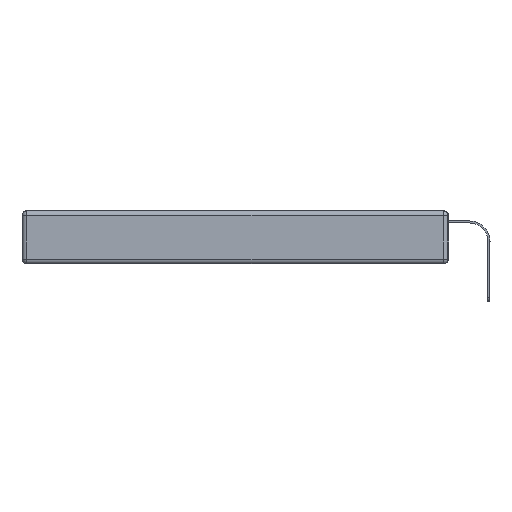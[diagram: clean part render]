
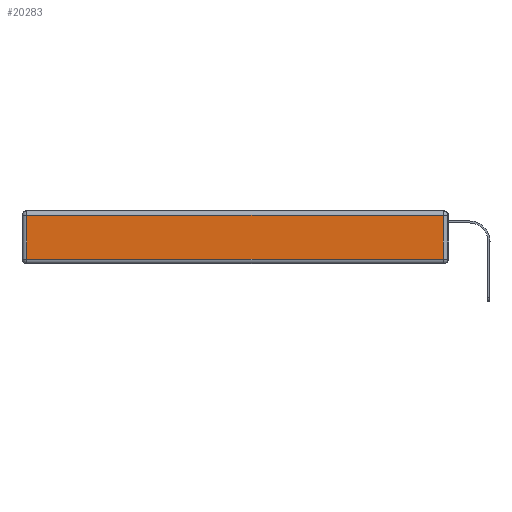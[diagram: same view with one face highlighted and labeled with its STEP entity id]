
A CAD part, left-side view. The second image highlights one B-rep face of the part: STEP entity #20283.
In plain terms, the highlighted planar face has unit normal (-1, 0, 0).
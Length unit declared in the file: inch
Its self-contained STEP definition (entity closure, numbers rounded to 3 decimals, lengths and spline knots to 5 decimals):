
#1440 = ORIENTED_EDGE ( 'NONE', *, *, #4398, .T. ) ;
#2004 = CARTESIAN_POINT ( 'NONE',  ( 0., 0.03, -0.03 ) ) ;
#2125 = VERTEX_POINT ( 'NONE', #2004 ) ;
#2507 = EDGE_CURVE ( 'NONE', #13487, #12943, #13361, .T. ) ;
#2826 = ORIENTED_EDGE ( 'NONE', *, *, #2507, .T. ) ;
#3901 = CARTESIAN_POINT ( 'NONE',  ( 0., 2.72, -0.343 ) ) ;
#3906 = VERTEX_POINT ( 'NONE', #17260 ) ;
#4398 = EDGE_CURVE ( 'NONE', #3906, #2125, #18825, .T. ) ;
#4701 = DIRECTION ( 'NONE',  ( 0., 0., 1. ) ) ;
#6167 = EDGE_LOOP ( 'NONE', ( #6197, #1440, #10350, #2826 ) ) ;
#6171 = LINE ( 'NONE', #14358, #8982 ) ;
#6197 = ORIENTED_EDGE ( 'NONE', *, *, #20880, .T. ) ;
#6198 = CARTESIAN_POINT ( 'NONE',  ( 0., 0., -0.343 ) ) ;
#7205 = DIRECTION ( 'NONE',  ( 0., -1., 0. ) ) ;
#8725 = CARTESIAN_POINT ( 'NONE',  ( 0., 0., -0.313 ) ) ;
#8902 = CARTESIAN_POINT ( 'NONE',  ( 0., 2.72, -0.03 ) ) ;
#8982 = VECTOR ( 'NONE', #14465, 39.37008 ) ;
#10042 = VECTOR ( 'NONE', #12471, 39.37008 ) ;
#10350 = ORIENTED_EDGE ( 'NONE', *, *, #18829, .T. ) ;
#10643 = CARTESIAN_POINT ( 'NONE',  ( 0., 0.03, -0.343 ) ) ;
#11172 = PLANE ( 'NONE',  #18253 ) ;
#12042 = CARTESIAN_POINT ( 'NONE',  ( 0., 2.72, -0.313 ) ) ;
#12471 = DIRECTION ( 'NONE',  ( 0., 0., 1. ) ) ;
#12766 = FACE_OUTER_BOUND ( 'NONE', #6167, .T. ) ;
#12943 = VERTEX_POINT ( 'NONE', #12042 ) ;
#13342 = VECTOR ( 'NONE', #15405, 39.37008 ) ;
#13361 = LINE ( 'NONE', #3901, #13342 ) ;
#13487 = VERTEX_POINT ( 'NONE', #8902 ) ;
#14358 = CARTESIAN_POINT ( 'NONE',  ( 0., 2.75, -0.03 ) ) ;
#14465 = DIRECTION ( 'NONE',  ( 0., 1., 0. ) ) ;
#15177 = VECTOR ( 'NONE', #7205, 39.37008 ) ;
#15405 = DIRECTION ( 'NONE',  ( 0., 0., -1. ) ) ;
#17260 = CARTESIAN_POINT ( 'NONE',  ( 0., 0.03, -0.313 ) ) ;
#17731 = DIRECTION ( 'NONE',  ( -1., 0., 0. ) ) ;
#18253 = AXIS2_PLACEMENT_3D ( 'NONE', #6198, #17731, #4701 ) ;
#18615 = LINE ( 'NONE', #8725, #15177 ) ;
#18825 = LINE ( 'NONE', #10643, #10042 ) ;
#18829 = EDGE_CURVE ( 'NONE', #2125, #13487, #6171, .T. ) ;
#20283 = ADVANCED_FACE ( 'NONE', ( #12766 ), #11172, .T. ) ;
#20880 = EDGE_CURVE ( 'NONE', #12943, #3906, #18615, .T. ) ;
